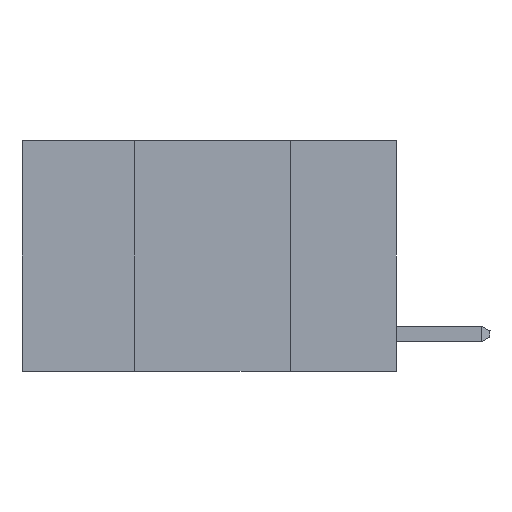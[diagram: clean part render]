
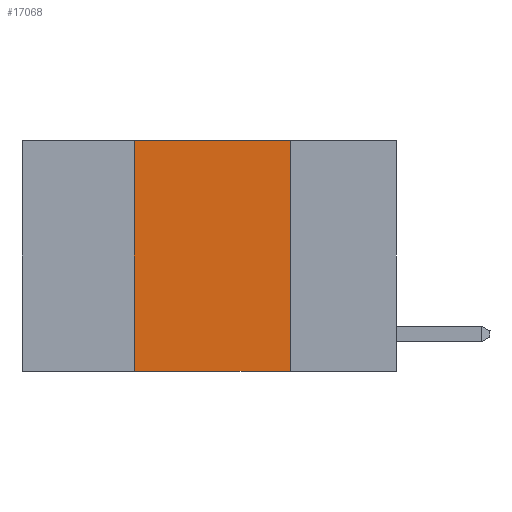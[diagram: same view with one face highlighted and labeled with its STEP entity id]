
A CAD part, left-side view. The second image highlights one B-rep face of the part: STEP entity #17068.
In plain terms, the highlighted planar face has unit normal (-1, 0, 0).
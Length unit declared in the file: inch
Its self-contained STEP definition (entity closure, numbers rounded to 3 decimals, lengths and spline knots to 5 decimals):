
#252 = LINE ( 'NONE', #6351, #8048 ) ;
#544 = DIRECTION ( 'NONE',  ( 0., 0., -1. ) ) ;
#592 = CARTESIAN_POINT ( 'NONE',  ( 0., 0.17, -0.37 ) ) ;
#625 = ORIENTED_EDGE ( 'NONE', *, *, #6369, .F. ) ;
#1166 = CARTESIAN_POINT ( 'NONE',  ( 0., 0.42, 0. ) ) ;
#2519 = CARTESIAN_POINT ( 'NONE',  ( 0., 0.6, -0.37 ) ) ;
#2670 = VERTEX_POINT ( 'NONE', #25635 ) ;
#5541 = DIRECTION ( 'NONE',  ( 0., 0., 1. ) ) ;
#6305 = VERTEX_POINT ( 'NONE', #20635 ) ;
#6351 = CARTESIAN_POINT ( 'NONE',  ( 0., 0.17, 0. ) ) ;
#6369 = EDGE_CURVE ( 'NONE', #6305, #2670, #18731, .T. ) ;
#6651 = ORIENTED_EDGE ( 'NONE', *, *, #14988, .F. ) ;
#6869 = FACE_OUTER_BOUND ( 'NONE', #15363, .T. ) ;
#8048 = VECTOR ( 'NONE', #26653, 39.37008 ) ;
#9344 = PLANE ( 'NONE',  #27101 ) ;
#9539 = CARTESIAN_POINT ( 'NONE',  ( 0., 0.6, 0. ) ) ;
#10159 = ORIENTED_EDGE ( 'NONE', *, *, #13673, .T. ) ;
#12308 = LINE ( 'NONE', #1166, #17291 ) ;
#12674 = VECTOR ( 'NONE', #14210, 39.37008 ) ;
#12754 = VECTOR ( 'NONE', #23125, 39.37008 ) ;
#13480 = LINE ( 'NONE', #2519, #12754 ) ;
#13673 = EDGE_CURVE ( 'NONE', #24009, #24301, #13480, .T. ) ;
#14210 = DIRECTION ( 'NONE',  ( 0., -1., 0. ) ) ;
#14988 = EDGE_CURVE ( 'NONE', #24009, #6305, #12308, .T. ) ;
#15363 = EDGE_LOOP ( 'NONE', ( #24518, #625, #6651, #10159 ) ) ;
#17068 = ADVANCED_FACE ( 'NONE', ( #6869 ), #9344, .F. ) ;
#17291 = VECTOR ( 'NONE', #5541, 39.37008 ) ;
#18731 = LINE ( 'NONE', #20927, #12674 ) ;
#20635 = CARTESIAN_POINT ( 'NONE',  ( 0., 0.42, 0. ) ) ;
#20927 = CARTESIAN_POINT ( 'NONE',  ( 0., 0.6, 0. ) ) ;
#22350 = CARTESIAN_POINT ( 'NONE',  ( 0., 0.42, -0.37 ) ) ;
#23125 = DIRECTION ( 'NONE',  ( 0., -1., 0. ) ) ;
#24009 = VERTEX_POINT ( 'NONE', #22350 ) ;
#24301 = VERTEX_POINT ( 'NONE', #592 ) ;
#24518 = ORIENTED_EDGE ( 'NONE', *, *, #27455, .F. ) ;
#25190 = DIRECTION ( 'NONE',  ( 1., 0., 0. ) ) ;
#25635 = CARTESIAN_POINT ( 'NONE',  ( 0., 0.17, 0. ) ) ;
#26653 = DIRECTION ( 'NONE',  ( 0., 0., -1. ) ) ;
#27101 = AXIS2_PLACEMENT_3D ( 'NONE', #9539, #25190, #544 ) ;
#27455 = EDGE_CURVE ( 'NONE', #2670, #24301, #252, .T. ) ;
